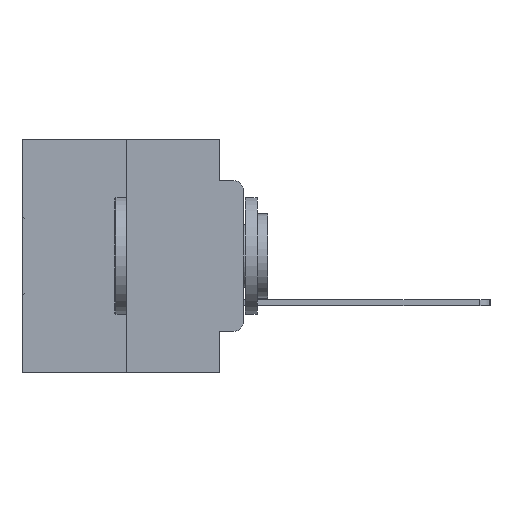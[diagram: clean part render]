
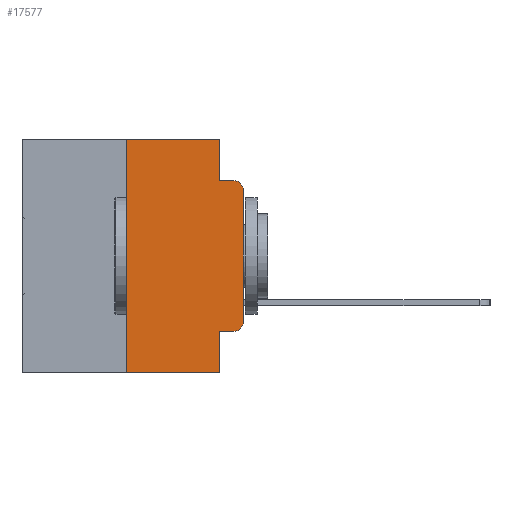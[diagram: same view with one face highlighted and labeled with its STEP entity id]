
A CAD part, left-side view. The second image highlights one B-rep face of the part: STEP entity #17577.
In plain terms, the highlighted planar face has unit normal (-1, 0, 0).
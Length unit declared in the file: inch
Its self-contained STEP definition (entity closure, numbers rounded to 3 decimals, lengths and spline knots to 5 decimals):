
#168 = AXIS2_PLACEMENT_3D ( 'NONE', #9565, #29161, #14554 ) ;
#309 = VERTEX_POINT ( 'NONE', #26016 ) ;
#594 = CARTESIAN_POINT ( 'NONE',  ( 0., 0.051, 0. ) ) ;
#621 = ORIENTED_EDGE ( 'NONE', *, *, #31562, .T. ) ;
#636 = EDGE_CURVE ( 'NONE', #27942, #15775, #6252, .T. ) ;
#724 = LINE ( 'NONE', #27717, #18978 ) ;
#828 = LINE ( 'NONE', #18626, #26395 ) ;
#1275 = VERTEX_POINT ( 'NONE', #14220 ) ;
#1276 = EDGE_CURVE ( 'NONE', #31767, #9241, #724, .T. ) ;
#1669 = VECTOR ( 'NONE', #13189, 39.37008 ) ;
#2275 = LINE ( 'NONE', #26329, #22718 ) ;
#3599 = CARTESIAN_POINT ( 'NONE',  ( 0., 0.25, 0. ) ) ;
#4512 = VECTOR ( 'NONE', #21707, 39.37008 ) ;
#4869 = CARTESIAN_POINT ( 'NONE',  ( 0., 0., -0.1085 ) ) ;
#5869 = CARTESIAN_POINT ( 'NONE',  ( 0., 0., 0. ) ) ;
#6012 = CARTESIAN_POINT ( 'NONE',  ( 0., 0.02, -0.1085 ) ) ;
#6252 = LINE ( 'NONE', #5869, #12142 ) ;
#6498 = ORIENTED_EDGE ( 'NONE', *, *, #1276, .T. ) ;
#6884 = CARTESIAN_POINT ( 'NONE',  ( 0., 0.473, 0. ) ) ;
#7000 = CARTESIAN_POINT ( 'NONE',  ( 0., 0.051, -0.4115 ) ) ;
#7275 = CARTESIAN_POINT ( 'NONE',  ( 0., 0.02, -0.0885 ) ) ;
#7975 = EDGE_CURVE ( 'NONE', #31767, #1275, #9118, .T. ) ;
#8542 = DIRECTION ( 'NONE',  ( 0., 0., -1. ) ) ;
#9118 = LINE ( 'NONE', #594, #1669 ) ;
#9241 = VERTEX_POINT ( 'NONE', #26743 ) ;
#9565 = CARTESIAN_POINT ( 'NONE',  ( 0., 0.473, 0. ) ) ;
#9670 = EDGE_CURVE ( 'NONE', #11055, #16761, #13406, .T. ) ;
#9976 = VERTEX_POINT ( 'NONE', #7275 ) ;
#10498 = CARTESIAN_POINT ( 'NONE',  ( 0., 0.051, 0. ) ) ;
#11055 = VERTEX_POINT ( 'NONE', #16668 ) ;
#11349 = EDGE_CURVE ( 'NONE', #22721, #309, #15585, .T. ) ;
#11790 = DIRECTION ( 'NONE',  ( 0., -1., 0. ) ) ;
#12086 = PLANE ( 'NONE',  #168 ) ;
#12142 = VECTOR ( 'NONE', #25793, 39.37008 ) ;
#12688 = DIRECTION ( 'NONE',  ( 0., -1., 0. ) ) ;
#12906 = CIRCLE ( 'NONE', #24147, 0.02 ) ;
#13189 = DIRECTION ( 'NONE',  ( 0., 0., -1. ) ) ;
#13406 = LINE ( 'NONE', #3599, #27194 ) ;
#13801 = DIRECTION ( 'NONE',  ( -1., 0., 0. ) ) ;
#14220 = CARTESIAN_POINT ( 'NONE',  ( 0., 0.051, -0.5 ) ) ;
#14554 = DIRECTION ( 'NONE',  ( 0., 0., -1. ) ) ;
#14579 = EDGE_LOOP ( 'NONE', ( #14668, #16956, #20019, #15072, #21585, #28055, #23094, #29569, #6498, #621 ) ) ;
#14668 = ORIENTED_EDGE ( 'NONE', *, *, #636, .T. ) ;
#15072 = ORIENTED_EDGE ( 'NONE', *, *, #11349, .F. ) ;
#15585 = LINE ( 'NONE', #10498, #21347 ) ;
#15659 = CARTESIAN_POINT ( 'NONE',  ( 0., 0.051, 0. ) ) ;
#15775 = VERTEX_POINT ( 'NONE', #4869 ) ;
#16668 = CARTESIAN_POINT ( 'NONE',  ( 0., 0.25, -0.5 ) ) ;
#16761 = VERTEX_POINT ( 'NONE', #30931 ) ;
#16956 = ORIENTED_EDGE ( 'NONE', *, *, #24515, .T. ) ;
#17577 = ADVANCED_FACE ( 'NONE', ( #28764 ), #12086, .F. ) ;
#17921 = DIRECTION ( 'NONE',  ( 0., 0., -1. ) ) ;
#18470 = LINE ( 'NONE', #6884, #4512 ) ;
#18626 = CARTESIAN_POINT ( 'NONE',  ( 0., 0.051, -0.0885 ) ) ;
#18978 = VECTOR ( 'NONE', #12688, 39.37008 ) ;
#20019 = ORIENTED_EDGE ( 'NONE', *, *, #22853, .F. ) ;
#21347 = VECTOR ( 'NONE', #17921, 39.37008 ) ;
#21585 = ORIENTED_EDGE ( 'NONE', *, *, #26394, .F. ) ;
#21650 = EDGE_CURVE ( 'NONE', #11055, #1275, #2275, .T. ) ;
#21707 = DIRECTION ( 'NONE',  ( 0., -1., 0. ) ) ;
#22533 = AXIS2_PLACEMENT_3D ( 'NONE', #6012, #23287, #8542 ) ;
#22718 = VECTOR ( 'NONE', #28736, 39.37008 ) ;
#22721 = VERTEX_POINT ( 'NONE', #15659 ) ;
#22853 = EDGE_CURVE ( 'NONE', #309, #9976, #828, .T. ) ;
#23094 = ORIENTED_EDGE ( 'NONE', *, *, #21650, .T. ) ;
#23287 = DIRECTION ( 'NONE',  ( -1., 0., 0. ) ) ;
#23314 = CARTESIAN_POINT ( 'NONE',  ( 0., 0., -0.3915 ) ) ;
#23377 = DIRECTION ( 'NONE',  ( 0., 0., 1. ) ) ;
#24147 = AXIS2_PLACEMENT_3D ( 'NONE', #28424, #13801, #30843 ) ;
#24515 = EDGE_CURVE ( 'NONE', #15775, #9976, #27412, .T. ) ;
#25793 = DIRECTION ( 'NONE',  ( 0., 0., 1. ) ) ;
#26016 = CARTESIAN_POINT ( 'NONE',  ( 0., 0.051, -0.0885 ) ) ;
#26329 = CARTESIAN_POINT ( 'NONE',  ( 0., 0.473, -0.5 ) ) ;
#26394 = EDGE_CURVE ( 'NONE', #16761, #22721, #18470, .T. ) ;
#26395 = VECTOR ( 'NONE', #11790, 39.37008 ) ;
#26743 = CARTESIAN_POINT ( 'NONE',  ( 0., 0.02, -0.4115 ) ) ;
#27194 = VECTOR ( 'NONE', #23377, 39.37008 ) ;
#27412 = CIRCLE ( 'NONE', #22533, 0.02 ) ;
#27717 = CARTESIAN_POINT ( 'NONE',  ( 0., 0.051, -0.4115 ) ) ;
#27942 = VERTEX_POINT ( 'NONE', #23314 ) ;
#28055 = ORIENTED_EDGE ( 'NONE', *, *, #9670, .F. ) ;
#28424 = CARTESIAN_POINT ( 'NONE',  ( 0., 0.02, -0.3915 ) ) ;
#28736 = DIRECTION ( 'NONE',  ( 0., -1., 0. ) ) ;
#28764 = FACE_OUTER_BOUND ( 'NONE', #14579, .T. ) ;
#29161 = DIRECTION ( 'NONE',  ( 1., 0., 0. ) ) ;
#29569 = ORIENTED_EDGE ( 'NONE', *, *, #7975, .F. ) ;
#30843 = DIRECTION ( 'NONE',  ( 0., 0., -1. ) ) ;
#30931 = CARTESIAN_POINT ( 'NONE',  ( 0., 0.25, 0. ) ) ;
#31562 = EDGE_CURVE ( 'NONE', #9241, #27942, #12906, .T. ) ;
#31767 = VERTEX_POINT ( 'NONE', #7000 ) ;
